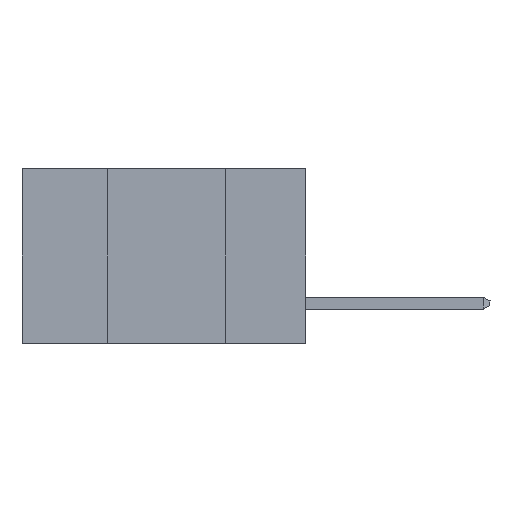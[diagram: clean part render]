
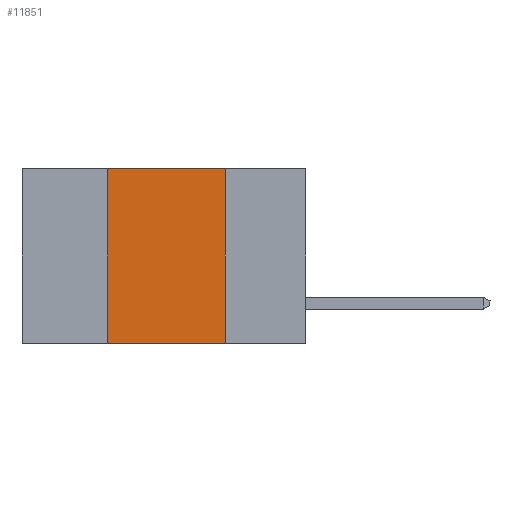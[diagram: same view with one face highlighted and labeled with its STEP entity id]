
A CAD part, left-side view. The second image highlights one B-rep face of the part: STEP entity #11851.
In plain terms, the highlighted planar face has unit normal (-1, 0, 0).
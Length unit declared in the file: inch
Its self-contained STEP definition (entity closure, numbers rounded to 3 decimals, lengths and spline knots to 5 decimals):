
#117 = VERTEX_POINT ( 'NONE', #18584 ) ;
#363 = CARTESIAN_POINT ( 'NONE',  ( 0., 0.6, 0. ) ) ;
#733 = AXIS2_PLACEMENT_3D ( 'NONE', #14459, #12757, #1446 ) ;
#1446 = DIRECTION ( 'NONE',  ( 0., 0., -1. ) ) ;
#1765 = VERTEX_POINT ( 'NONE', #21585 ) ;
#2115 = EDGE_CURVE ( 'NONE', #23716, #8069, #12478, .T. ) ;
#2737 = EDGE_CURVE ( 'NONE', #117, #1765, #22252, .T. ) ;
#3692 = DIRECTION ( 'NONE',  ( 0., -1., 0. ) ) ;
#5708 = ORIENTED_EDGE ( 'NONE', *, *, #21605, .F. ) ;
#5739 = DIRECTION ( 'NONE',  ( 0., -1., 0. ) ) ;
#7435 = CARTESIAN_POINT ( 'NONE',  ( 0., 0.6, -0.37 ) ) ;
#8069 = VERTEX_POINT ( 'NONE', #14090 ) ;
#10615 = EDGE_LOOP ( 'NONE', ( #21031, #5708, #21450, #13044 ) ) ;
#11241 = CARTESIAN_POINT ( 'NONE',  ( 0., 0.17, 0. ) ) ;
#11851 = ADVANCED_FACE ( 'NONE', ( #16437 ), #23493, .F. ) ;
#12049 = VECTOR ( 'NONE', #3692, 39.37008 ) ;
#12478 = LINE ( 'NONE', #20857, #13914 ) ;
#12757 = DIRECTION ( 'NONE',  ( 1., 0., 0. ) ) ;
#13044 = ORIENTED_EDGE ( 'NONE', *, *, #15175, .T. ) ;
#13914 = VECTOR ( 'NONE', #22534, 39.37008 ) ;
#14090 = CARTESIAN_POINT ( 'NONE',  ( 0., 0.17, -0.37 ) ) ;
#14459 = CARTESIAN_POINT ( 'NONE',  ( 0., 0.6, 0. ) ) ;
#14941 = CARTESIAN_POINT ( 'NONE',  ( 0., 0.42, 0. ) ) ;
#15175 = EDGE_CURVE ( 'NONE', #117, #8069, #22817, .T. ) ;
#16437 = FACE_OUTER_BOUND ( 'NONE', #10615, .T. ) ;
#18584 = CARTESIAN_POINT ( 'NONE',  ( 0., 0.42, -0.37 ) ) ;
#18797 = VECTOR ( 'NONE', #20524, 39.37008 ) ;
#19664 = VECTOR ( 'NONE', #5739, 39.37008 ) ;
#20524 = DIRECTION ( 'NONE',  ( 0., 0., 1. ) ) ;
#20857 = CARTESIAN_POINT ( 'NONE',  ( 0., 0.17, 0. ) ) ;
#21031 = ORIENTED_EDGE ( 'NONE', *, *, #2115, .F. ) ;
#21450 = ORIENTED_EDGE ( 'NONE', *, *, #2737, .F. ) ;
#21585 = CARTESIAN_POINT ( 'NONE',  ( 0., 0.42, 0. ) ) ;
#21605 = EDGE_CURVE ( 'NONE', #1765, #23716, #21859, .T. ) ;
#21859 = LINE ( 'NONE', #363, #12049 ) ;
#22252 = LINE ( 'NONE', #14941, #18797 ) ;
#22534 = DIRECTION ( 'NONE',  ( 0., 0., -1. ) ) ;
#22817 = LINE ( 'NONE', #7435, #19664 ) ;
#23493 = PLANE ( 'NONE',  #733 ) ;
#23716 = VERTEX_POINT ( 'NONE', #11241 ) ;
